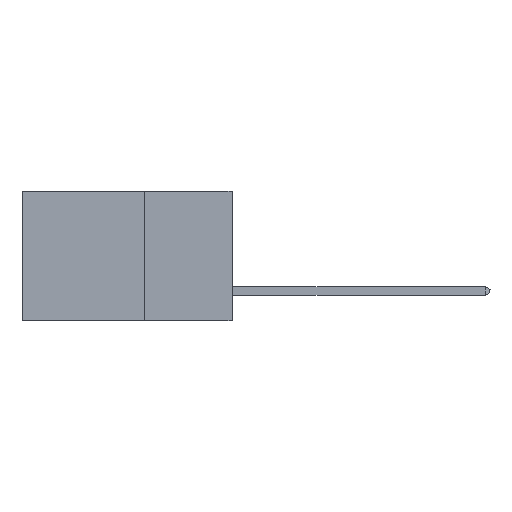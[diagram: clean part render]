
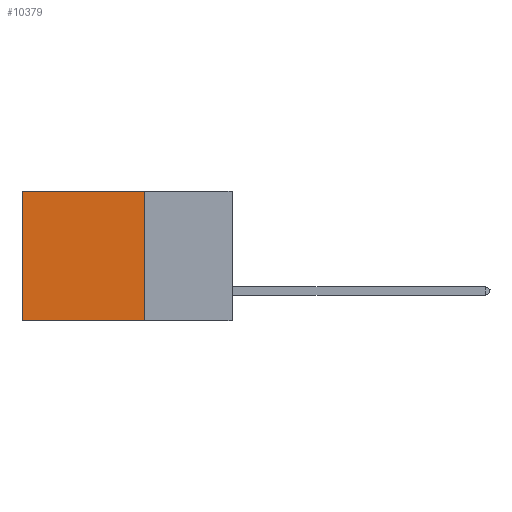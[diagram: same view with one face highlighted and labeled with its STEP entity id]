
A CAD part, left-side view. The second image highlights one B-rep face of the part: STEP entity #10379.
In plain terms, the highlighted planar face has unit normal (-1, 0, 0).
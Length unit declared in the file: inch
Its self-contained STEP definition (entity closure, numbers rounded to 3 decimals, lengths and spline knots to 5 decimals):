
#1012 = CARTESIAN_POINT ( 'NONE',  ( 0.2875, 0.6, 0. ) ) ;
#1211 = EDGE_CURVE ( 'NONE', #16760, #30063, #16807, .T. ) ;
#2685 = CARTESIAN_POINT ( 'NONE',  ( 0.2875, 0.25, 0. ) ) ;
#3655 = EDGE_CURVE ( 'NONE', #16760, #34466, #33840, .T. ) ;
#5140 = DIRECTION ( 'NONE',  ( 0., 1., 0. ) ) ;
#8671 = CARTESIAN_POINT ( 'NONE',  ( 0.2875, 0.25, -0.37 ) ) ;
#9052 = PLANE ( 'NONE',  #31062 ) ;
#9365 = DIRECTION ( 'NONE',  ( 1., 0., 0. ) ) ;
#10379 = ADVANCED_FACE ( 'NONE', ( #41985 ), #9052, .F. ) ;
#10951 = ORIENTED_EDGE ( 'NONE', *, *, #36523, .F. ) ;
#11400 = DIRECTION ( 'NONE',  ( 0., 0., -1. ) ) ;
#16760 = VERTEX_POINT ( 'NONE', #38873 ) ;
#16807 = LINE ( 'NONE', #30922, #22516 ) ;
#19289 = CARTESIAN_POINT ( 'NONE',  ( 0.2875, 0.6, 0. ) ) ;
#20354 = CARTESIAN_POINT ( 'NONE',  ( 0.2875, 0.25, 0. ) ) ;
#20710 = ORIENTED_EDGE ( 'NONE', *, *, #30295, .T. ) ;
#22516 = VECTOR ( 'NONE', #11400, 39.37008 ) ;
#22760 = DIRECTION ( 'NONE',  ( 0., 0., -1. ) ) ;
#24107 = DIRECTION ( 'NONE',  ( 0., 1., 0. ) ) ;
#30063 = VERTEX_POINT ( 'NONE', #34299 ) ;
#30295 = EDGE_CURVE ( 'NONE', #34466, #41049, #32919, .T. ) ;
#30338 = DIRECTION ( 'NONE',  ( 0., 0., -1. ) ) ;
#30922 = CARTESIAN_POINT ( 'NONE',  ( 0.2875, 0.25, 0. ) ) ;
#31062 = AXIS2_PLACEMENT_3D ( 'NONE', #2685, #9365, #22760 ) ;
#32098 = ORIENTED_EDGE ( 'NONE', *, *, #1211, .F. ) ;
#32844 = CARTESIAN_POINT ( 'NONE',  ( 0.2875, 0.6, -0.37 ) ) ;
#32919 = LINE ( 'NONE', #19289, #39709 ) ;
#33840 = LINE ( 'NONE', #20354, #36505 ) ;
#34299 = CARTESIAN_POINT ( 'NONE',  ( 0.2875, 0.25, -0.37 ) ) ;
#34417 = LINE ( 'NONE', #8671, #41786 ) ;
#34466 = VERTEX_POINT ( 'NONE', #1012 ) ;
#34734 = ORIENTED_EDGE ( 'NONE', *, *, #3655, .T. ) ;
#36505 = VECTOR ( 'NONE', #24107, 39.37008 ) ;
#36523 = EDGE_CURVE ( 'NONE', #30063, #41049, #34417, .T. ) ;
#38873 = CARTESIAN_POINT ( 'NONE',  ( 0.2875, 0.25, 0. ) ) ;
#39709 = VECTOR ( 'NONE', #30338, 39.37008 ) ;
#41049 = VERTEX_POINT ( 'NONE', #32844 ) ;
#41786 = VECTOR ( 'NONE', #5140, 39.37008 ) ;
#41965 = EDGE_LOOP ( 'NONE', ( #20710, #10951, #32098, #34734 ) ) ;
#41985 = FACE_OUTER_BOUND ( 'NONE', #41965, .T. ) ;
